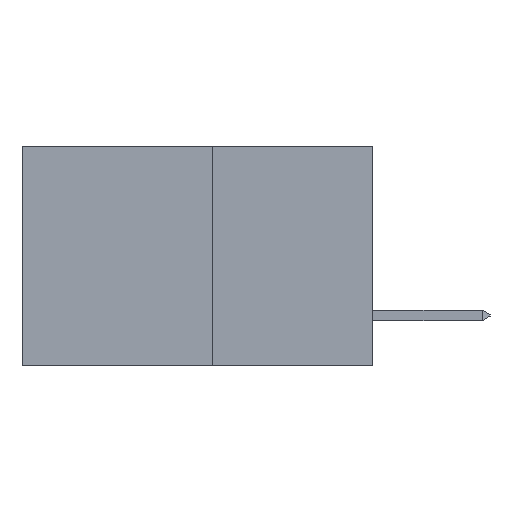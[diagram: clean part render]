
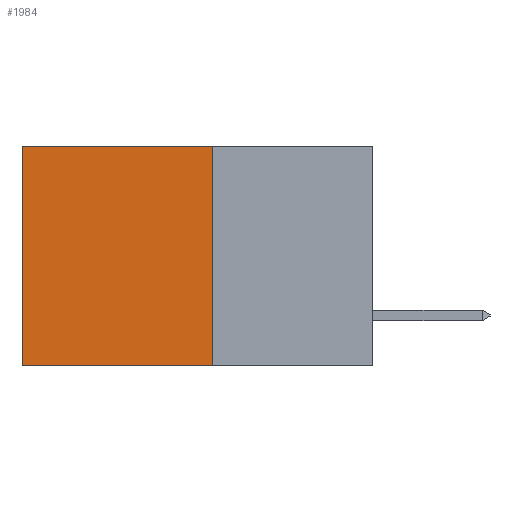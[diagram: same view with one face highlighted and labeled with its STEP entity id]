
A CAD part, left-side view. The second image highlights one B-rep face of the part: STEP entity #1984.
In plain terms, the highlighted planar face has unit normal (-1, 0, 0).
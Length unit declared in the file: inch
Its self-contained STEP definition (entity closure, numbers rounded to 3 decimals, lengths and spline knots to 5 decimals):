
#114 = EDGE_CURVE ( 'NONE', #7258, #306, #11868, .T. ) ;
#304 = CARTESIAN_POINT ( 'NONE',  ( 0.277, 0.59, 0. ) ) ;
#306 = VERTEX_POINT ( 'NONE', #5288 ) ;
#740 = EDGE_CURVE ( 'NONE', #10888, #306, #1946, .T. ) ;
#832 = DIRECTION ( 'NONE',  ( 0., 1., 0. ) ) ;
#1449 = LINE ( 'NONE', #10783, #6803 ) ;
#1946 = LINE ( 'NONE', #7698, #4294 ) ;
#1984 = ADVANCED_FACE ( 'NONE', ( #11214 ), #3869, .F. ) ;
#2863 = CARTESIAN_POINT ( 'NONE',  ( 0.277, 0.27, 0. ) ) ;
#3149 = CARTESIAN_POINT ( 'NONE',  ( 0.277, 0.27, 0. ) ) ;
#3206 = ORIENTED_EDGE ( 'NONE', *, *, #6538, .F. ) ;
#3826 = VECTOR ( 'NONE', #11213, 39.37008 ) ;
#3869 = PLANE ( 'NONE',  #5225 ) ;
#4069 = VECTOR ( 'NONE', #832, 39.37008 ) ;
#4294 = VECTOR ( 'NONE', #6508, 39.37008 ) ;
#4653 = ORIENTED_EDGE ( 'NONE', *, *, #740, .F. ) ;
#5052 = EDGE_LOOP ( 'NONE', ( #5542, #4653, #3206, #6855 ) ) ;
#5225 = AXIS2_PLACEMENT_3D ( 'NONE', #8164, #6848, #6122 ) ;
#5288 = CARTESIAN_POINT ( 'NONE',  ( 0.277, 0.59, -0.37 ) ) ;
#5467 = VERTEX_POINT ( 'NONE', #3149 ) ;
#5542 = ORIENTED_EDGE ( 'NONE', *, *, #114, .T. ) ;
#6122 = DIRECTION ( 'NONE',  ( 0., 0., -1. ) ) ;
#6508 = DIRECTION ( 'NONE',  ( 0., 1., 0. ) ) ;
#6538 = EDGE_CURVE ( 'NONE', #5467, #10888, #1449, .T. ) ;
#6803 = VECTOR ( 'NONE', #8870, 39.37008 ) ;
#6848 = DIRECTION ( 'NONE',  ( 1., 0., 0. ) ) ;
#6855 = ORIENTED_EDGE ( 'NONE', *, *, #12468, .T. ) ;
#7258 = VERTEX_POINT ( 'NONE', #304 ) ;
#7603 = CARTESIAN_POINT ( 'NONE',  ( 0.277, 0.27, -0.37 ) ) ;
#7698 = CARTESIAN_POINT ( 'NONE',  ( 0.277, 0.27, -0.37 ) ) ;
#8164 = CARTESIAN_POINT ( 'NONE',  ( 0.277, 0.27, -0.37 ) ) ;
#8870 = DIRECTION ( 'NONE',  ( 0., 0., -1. ) ) ;
#8888 = CARTESIAN_POINT ( 'NONE',  ( 0.277, 0.59, -0.37 ) ) ;
#10783 = CARTESIAN_POINT ( 'NONE',  ( 0.277, 0.27, -0.37 ) ) ;
#10888 = VERTEX_POINT ( 'NONE', #7603 ) ;
#11213 = DIRECTION ( 'NONE',  ( 0., 0., -1. ) ) ;
#11214 = FACE_OUTER_BOUND ( 'NONE', #5052, .T. ) ;
#11782 = LINE ( 'NONE', #2863, #4069 ) ;
#11868 = LINE ( 'NONE', #8888, #3826 ) ;
#12468 = EDGE_CURVE ( 'NONE', #5467, #7258, #11782, .T. ) ;
